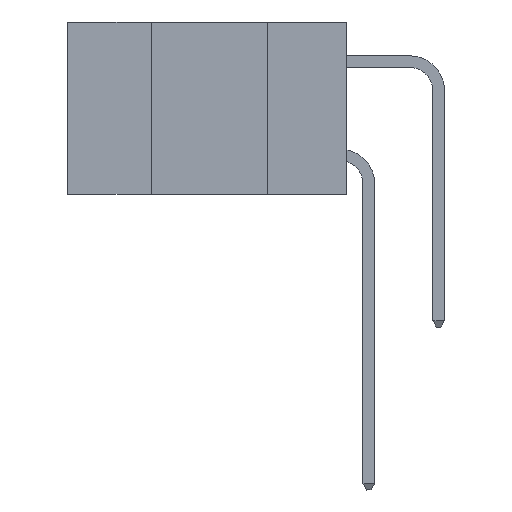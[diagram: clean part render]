
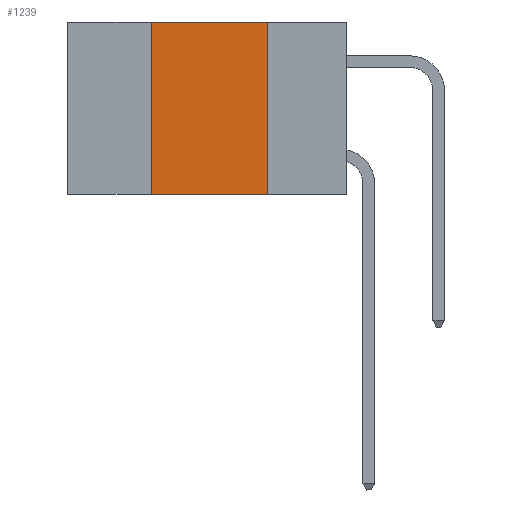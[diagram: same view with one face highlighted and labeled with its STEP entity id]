
A CAD part, left-side view. The second image highlights one B-rep face of the part: STEP entity #1239.
In plain terms, the highlighted planar face has unit normal (-1, 0, 0).
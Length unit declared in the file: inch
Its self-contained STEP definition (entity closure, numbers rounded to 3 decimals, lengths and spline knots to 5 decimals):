
#607 = VECTOR ( 'NONE', #8829, 39.37008 ) ;
#1061 = EDGE_CURVE ( 'NONE', #12624, #10025, #6257, .T. ) ;
#1184 = CARTESIAN_POINT ( 'NONE',  ( 0., 0.42, 0. ) ) ;
#1239 = ADVANCED_FACE ( 'NONE', ( #4588 ), #12910, .F. ) ;
#1524 = CARTESIAN_POINT ( 'NONE',  ( 0., 0.17, -0.37 ) ) ;
#1685 = CARTESIAN_POINT ( 'NONE',  ( 0., 0.6, 0. ) ) ;
#2075 = VERTEX_POINT ( 'NONE', #12341 ) ;
#2225 = DIRECTION ( 'NONE',  ( 0., 0., -1. ) ) ;
#2541 = VECTOR ( 'NONE', #3171, 39.37008 ) ;
#2762 = DIRECTION ( 'NONE',  ( 0., -1., 0. ) ) ;
#2962 = ORIENTED_EDGE ( 'NONE', *, *, #1061, .F. ) ;
#3171 = DIRECTION ( 'NONE',  ( 0., 0., 1. ) ) ;
#4028 = CARTESIAN_POINT ( 'NONE',  ( 0., 0.17, 0. ) ) ;
#4588 = FACE_OUTER_BOUND ( 'NONE', #5900, .T. ) ;
#4833 = DIRECTION ( 'NONE',  ( 1., 0., 0. ) ) ;
#5305 = CARTESIAN_POINT ( 'NONE',  ( 0., 0.17, 0. ) ) ;
#5435 = EDGE_CURVE ( 'NONE', #2075, #10025, #13152, .T. ) ;
#5900 = EDGE_LOOP ( 'NONE', ( #2962, #7472, #10761, #6083 ) ) ;
#6083 = ORIENTED_EDGE ( 'NONE', *, *, #5435, .T. ) ;
#6257 = LINE ( 'NONE', #5305, #9298 ) ;
#6712 = AXIS2_PLACEMENT_3D ( 'NONE', #1685, #4833, #8843 ) ;
#6793 = VECTOR ( 'NONE', #2762, 39.37008 ) ;
#6938 = CARTESIAN_POINT ( 'NONE',  ( 0., 0.6, 0. ) ) ;
#7424 = EDGE_CURVE ( 'NONE', #12504, #12624, #11426, .T. ) ;
#7472 = ORIENTED_EDGE ( 'NONE', *, *, #7424, .F. ) ;
#8080 = LINE ( 'NONE', #1184, #2541 ) ;
#8829 = DIRECTION ( 'NONE',  ( 0., -1., 0. ) ) ;
#8843 = DIRECTION ( 'NONE',  ( 0., 0., -1. ) ) ;
#9122 = EDGE_CURVE ( 'NONE', #2075, #12504, #8080, .T. ) ;
#9298 = VECTOR ( 'NONE', #2225, 39.37008 ) ;
#10025 = VERTEX_POINT ( 'NONE', #1524 ) ;
#10689 = CARTESIAN_POINT ( 'NONE',  ( 0., 0.6, -0.37 ) ) ;
#10761 = ORIENTED_EDGE ( 'NONE', *, *, #9122, .F. ) ;
#11426 = LINE ( 'NONE', #6938, #6793 ) ;
#12341 = CARTESIAN_POINT ( 'NONE',  ( 0., 0.42, -0.37 ) ) ;
#12504 = VERTEX_POINT ( 'NONE', #12915 ) ;
#12624 = VERTEX_POINT ( 'NONE', #4028 ) ;
#12910 = PLANE ( 'NONE',  #6712 ) ;
#12915 = CARTESIAN_POINT ( 'NONE',  ( 0., 0.42, 0. ) ) ;
#13152 = LINE ( 'NONE', #10689, #607 ) ;
